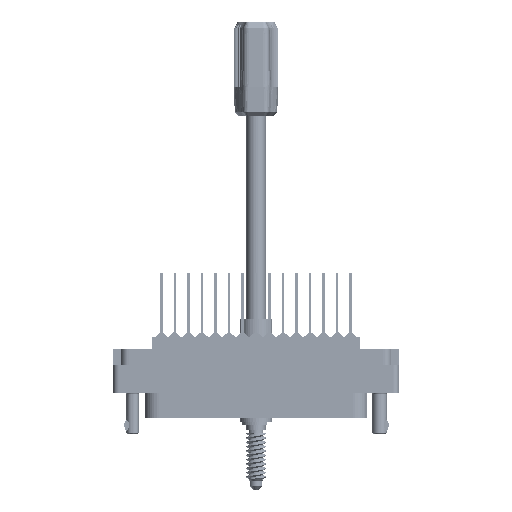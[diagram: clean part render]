
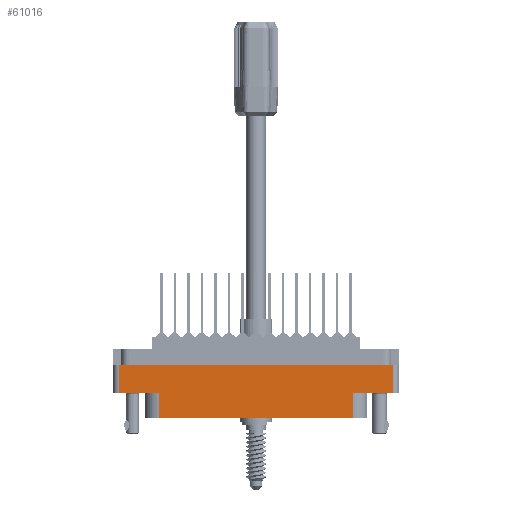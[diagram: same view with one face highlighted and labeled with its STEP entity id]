
A CAD part, front view. The second image highlights one B-rep face of the part: STEP entity #61016.
In plain terms, the highlighted planar face has unit normal (0, -1, 0).
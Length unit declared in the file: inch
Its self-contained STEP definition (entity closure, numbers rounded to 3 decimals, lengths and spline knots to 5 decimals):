
#1586 = DIRECTION ( 'NONE',  ( 0., 0., -1. ) ) ;
#5215 = EDGE_CURVE ( 'NONE', #12015, #33503, #17732, .T. ) ;
#5407 = DIRECTION ( 'NONE',  ( -1., 0., 0. ) ) ;
#5503 = VERTEX_POINT ( 'NONE', #27480 ) ;
#7088 = LINE ( 'NONE', #54131, #109918 ) ;
#8548 = CARTESIAN_POINT ( 'NONE',  ( 0.9315, -0.7625, -0.78 ) ) ;
#8806 = ORIENTED_EDGE ( 'NONE', *, *, #82755, .T. ) ;
#11971 = ORIENTED_EDGE ( 'NONE', *, *, #25062, .F. ) ;
#12015 = VERTEX_POINT ( 'NONE', #55057 ) ;
#12227 = VECTOR ( 'NONE', #5407, 39.37008 ) ;
#13837 = ORIENTED_EDGE ( 'NONE', *, *, #21195, .T. ) ;
#14311 = EDGE_LOOP ( 'NONE', ( #18278, #44233, #85822, #8806, #13837, #102163, #11971, #96223 ) ) ;
#16346 = EDGE_CURVE ( 'NONE', #5503, #57733, #79641, .T. ) ;
#17732 = LINE ( 'NONE', #99820, #97333 ) ;
#18278 = ORIENTED_EDGE ( 'NONE', *, *, #110769, .F. ) ;
#20475 = LINE ( 'NONE', #82459, #12227 ) ;
#21195 = EDGE_CURVE ( 'NONE', #56568, #34598, #54188, .T. ) ;
#25062 = EDGE_CURVE ( 'NONE', #12015, #67412, #20475, .T. ) ;
#26231 = DIRECTION ( 'NONE',  ( 1., 0., 0. ) ) ;
#27107 = CARTESIAN_POINT ( 'NONE',  ( -0.9315, -0.7625, -0.54 ) ) ;
#27480 = CARTESIAN_POINT ( 'NONE',  ( -1.313, -0.7625, -0.274 ) ) ;
#27803 = VERTEX_POINT ( 'NONE', #27107 ) ;
#33503 = VERTEX_POINT ( 'NONE', #85133 ) ;
#33988 = CARTESIAN_POINT ( 'NONE',  ( -0.9315, -0.7625, -0.78 ) ) ;
#34333 = VECTOR ( 'NONE', #44809, 39.37008 ) ;
#34598 = VERTEX_POINT ( 'NONE', #8548 ) ;
#38533 = EDGE_CURVE ( 'NONE', #57733, #27803, #113144, .T. ) ;
#39328 = PLANE ( 'NONE',  #65901 ) ;
#44233 = ORIENTED_EDGE ( 'NONE', *, *, #16346, .T. ) ;
#44809 = DIRECTION ( 'NONE',  ( 0., 0., 1. ) ) ;
#47711 = CARTESIAN_POINT ( 'NONE',  ( -1.313, -0.7625, -0.54 ) ) ;
#48187 = VECTOR ( 'NONE', #63581, 39.37008 ) ;
#52280 = CARTESIAN_POINT ( 'NONE',  ( -1.375, -0.7625, -0.78 ) ) ;
#54131 = CARTESIAN_POINT ( 'NONE',  ( -0.9315, -0.7625, -0.78 ) ) ;
#54188 = LINE ( 'NONE', #52280, #82985 ) ;
#55043 = DIRECTION ( 'NONE',  ( 1., 0., 0. ) ) ;
#55057 = CARTESIAN_POINT ( 'NONE',  ( 1.313, -0.7625, -0.54 ) ) ;
#55637 = CARTESIAN_POINT ( 'NONE',  ( -1.313, -0.7625, -0.78 ) ) ;
#56568 = VERTEX_POINT ( 'NONE', #33988 ) ;
#57733 = VERTEX_POINT ( 'NONE', #47711 ) ;
#58089 = DIRECTION ( 'NONE',  ( 0., 0., -1. ) ) ;
#61016 = ADVANCED_FACE ( 'NONE', ( #79182 ), #39328, .T. ) ;
#63581 = DIRECTION ( 'NONE',  ( 0., 0., -1. ) ) ;
#65756 = CARTESIAN_POINT ( 'NONE',  ( -1.375, -0.7625, -0.78 ) ) ;
#65901 = AXIS2_PLACEMENT_3D ( 'NONE', #65756, #110498, #58089 ) ;
#66464 = CARTESIAN_POINT ( 'NONE',  ( 0., -0.7625, -0.54 ) ) ;
#66587 = CARTESIAN_POINT ( 'NONE',  ( 0.9315, -0.7625, -0.54 ) ) ;
#67412 = VERTEX_POINT ( 'NONE', #66587 ) ;
#71615 = CARTESIAN_POINT ( 'NONE',  ( 0.9315, -0.7625, -0.54 ) ) ;
#76415 = EDGE_CURVE ( 'NONE', #34598, #67412, #109669, .T. ) ;
#79182 = FACE_OUTER_BOUND ( 'NONE', #14311, .T. ) ;
#79641 = LINE ( 'NONE', #55637, #48187 ) ;
#82459 = CARTESIAN_POINT ( 'NONE',  ( 0., -0.7625, -0.54 ) ) ;
#82550 = DIRECTION ( 'NONE',  ( 0., 0., 1. ) ) ;
#82755 = EDGE_CURVE ( 'NONE', #27803, #56568, #7088, .T. ) ;
#82985 = VECTOR ( 'NONE', #26231, 39.37008 ) ;
#85133 = CARTESIAN_POINT ( 'NONE',  ( 1.313, -0.7625, -0.274 ) ) ;
#85822 = ORIENTED_EDGE ( 'NONE', *, *, #38533, .T. ) ;
#86063 = LINE ( 'NONE', #107524, #99703 ) ;
#91312 = VECTOR ( 'NONE', #111622, 39.37008 ) ;
#96223 = ORIENTED_EDGE ( 'NONE', *, *, #5215, .T. ) ;
#97333 = VECTOR ( 'NONE', #82550, 39.37008 ) ;
#99703 = VECTOR ( 'NONE', #55043, 39.37008 ) ;
#99820 = CARTESIAN_POINT ( 'NONE',  ( 1.313, -0.7625, -0.78 ) ) ;
#102163 = ORIENTED_EDGE ( 'NONE', *, *, #76415, .T. ) ;
#107524 = CARTESIAN_POINT ( 'NONE',  ( 0., -0.7625, -0.274 ) ) ;
#109669 = LINE ( 'NONE', #71615, #34333 ) ;
#109918 = VECTOR ( 'NONE', #1586, 39.37008 ) ;
#110498 = DIRECTION ( 'NONE',  ( 0., -1., 0. ) ) ;
#110769 = EDGE_CURVE ( 'NONE', #5503, #33503, #86063, .T. ) ;
#111622 = DIRECTION ( 'NONE',  ( 1., 0., 0. ) ) ;
#113144 = LINE ( 'NONE', #66464, #91312 ) ;
